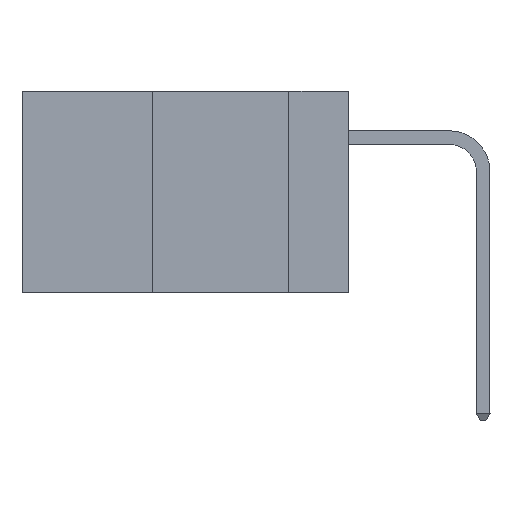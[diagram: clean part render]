
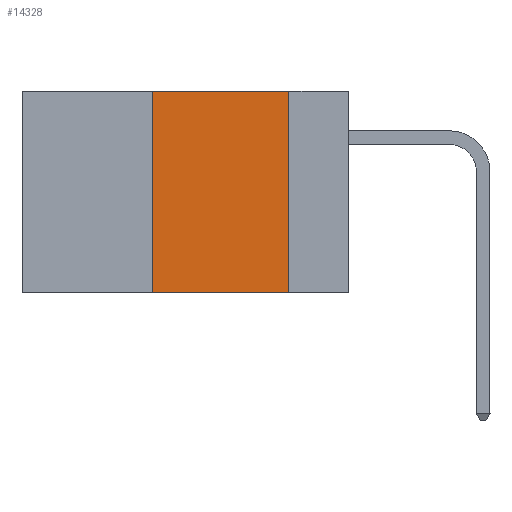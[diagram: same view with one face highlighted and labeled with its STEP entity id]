
A CAD part, left-side view. The second image highlights one B-rep face of the part: STEP entity #14328.
In plain terms, the highlighted planar face has unit normal (-1, 0, 0).
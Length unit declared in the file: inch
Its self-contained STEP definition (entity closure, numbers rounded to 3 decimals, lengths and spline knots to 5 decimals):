
#286 = CARTESIAN_POINT ( 'NONE',  ( 0., 0.11, -0.37 ) ) ;
#2121 = CARTESIAN_POINT ( 'NONE',  ( 0., 0.6, -0.37 ) ) ;
#3598 = CARTESIAN_POINT ( 'NONE',  ( 0., 0.36, -0.37 ) ) ;
#3787 = CARTESIAN_POINT ( 'NONE',  ( 0., 0.11, 0. ) ) ;
#4341 = EDGE_CURVE ( 'NONE', #33103, #26412, #34468, .T. ) ;
#6224 = CARTESIAN_POINT ( 'NONE',  ( 0., 0.6, 0. ) ) ;
#8761 = VERTEX_POINT ( 'NONE', #3598 ) ;
#9330 = FACE_OUTER_BOUND ( 'NONE', #14555, .T. ) ;
#11869 = ORIENTED_EDGE ( 'NONE', *, *, #4341, .F. ) ;
#14328 = ADVANCED_FACE ( 'NONE', ( #9330 ), #30776, .F. ) ;
#14555 = EDGE_LOOP ( 'NONE', ( #11869, #32714, #26424, #44865 ) ) ;
#21428 = VECTOR ( 'NONE', #30406, 39.37008 ) ;
#22475 = LINE ( 'NONE', #33434, #33219 ) ;
#23512 = DIRECTION ( 'NONE',  ( 0., 0., -1. ) ) ;
#24330 = DIRECTION ( 'NONE',  ( 1., 0., 0. ) ) ;
#26412 = VERTEX_POINT ( 'NONE', #286 ) ;
#26424 = ORIENTED_EDGE ( 'NONE', *, *, #35950, .F. ) ;
#26680 = LINE ( 'NONE', #2121, #39653 ) ;
#27066 = LINE ( 'NONE', #44955, #21428 ) ;
#27314 = CARTESIAN_POINT ( 'NONE',  ( 0., 0.11, 0. ) ) ;
#30406 = DIRECTION ( 'NONE',  ( 0., -1., 0. ) ) ;
#30776 = PLANE ( 'NONE',  #38623 ) ;
#31241 = DIRECTION ( 'NONE',  ( 0., 0., -1. ) ) ;
#32714 = ORIENTED_EDGE ( 'NONE', *, *, #44984, .F. ) ;
#33103 = VERTEX_POINT ( 'NONE', #3787 ) ;
#33219 = VECTOR ( 'NONE', #37006, 39.37008 ) ;
#33387 = VERTEX_POINT ( 'NONE', #34702 ) ;
#33434 = CARTESIAN_POINT ( 'NONE',  ( 0., 0.36, 0. ) ) ;
#34468 = LINE ( 'NONE', #27314, #45871 ) ;
#34702 = CARTESIAN_POINT ( 'NONE',  ( 0., 0.36, 0. ) ) ;
#35950 = EDGE_CURVE ( 'NONE', #8761, #33387, #22475, .T. ) ;
#36750 = EDGE_CURVE ( 'NONE', #8761, #26412, #26680, .T. ) ;
#37006 = DIRECTION ( 'NONE',  ( 0., 0., 1. ) ) ;
#38623 = AXIS2_PLACEMENT_3D ( 'NONE', #6224, #24330, #31241 ) ;
#39653 = VECTOR ( 'NONE', #45708, 39.37008 ) ;
#44865 = ORIENTED_EDGE ( 'NONE', *, *, #36750, .T. ) ;
#44955 = CARTESIAN_POINT ( 'NONE',  ( 0., 0.6, 0. ) ) ;
#44984 = EDGE_CURVE ( 'NONE', #33387, #33103, #27066, .T. ) ;
#45708 = DIRECTION ( 'NONE',  ( 0., -1., 0. ) ) ;
#45871 = VECTOR ( 'NONE', #23512, 39.37008 ) ;
